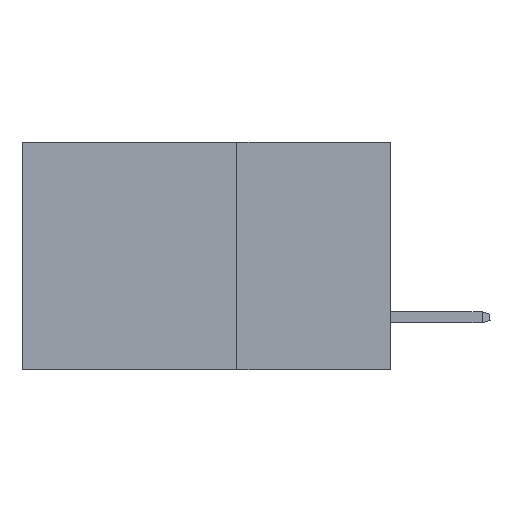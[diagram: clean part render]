
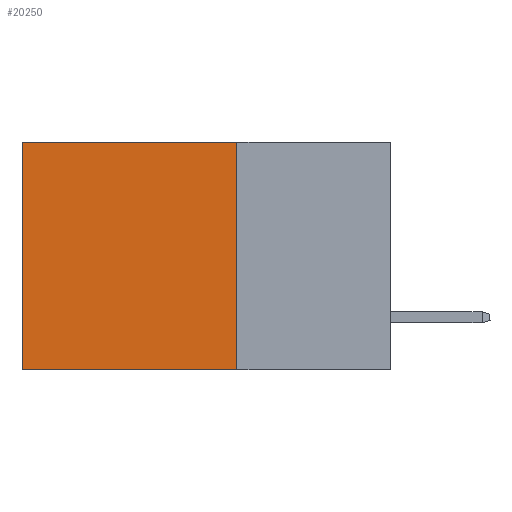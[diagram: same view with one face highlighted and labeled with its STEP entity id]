
A CAD part, left-side view. The second image highlights one B-rep face of the part: STEP entity #20250.
In plain terms, the highlighted planar face has unit normal (-1, 0, 0).
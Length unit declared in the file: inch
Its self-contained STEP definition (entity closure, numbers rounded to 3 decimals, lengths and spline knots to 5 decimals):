
#39 = ORIENTED_EDGE ( 'NONE', *, *, #12450, .F. ) ;
#1543 = CARTESIAN_POINT ( 'NONE',  ( 0.2875, 0.6, -0.37 ) ) ;
#7767 = LINE ( 'NONE', #8993, #19526 ) ;
#8753 = DIRECTION ( 'NONE',  ( 0., 0., -1. ) ) ;
#8993 = CARTESIAN_POINT ( 'NONE',  ( 0.2875, 0.25, 0. ) ) ;
#10341 = LINE ( 'NONE', #31055, #33421 ) ;
#11597 = ORIENTED_EDGE ( 'NONE', *, *, #26522, .T. ) ;
#12280 = DIRECTION ( 'NONE',  ( 0., 0., -1. ) ) ;
#12450 = EDGE_CURVE ( 'NONE', #19710, #16408, #22103, .T. ) ;
#13900 = CARTESIAN_POINT ( 'NONE',  ( 0.2875, 0.25, 0. ) ) ;
#15203 = PLANE ( 'NONE',  #25376 ) ;
#16408 = VERTEX_POINT ( 'NONE', #1543 ) ;
#16496 = VECTOR ( 'NONE', #16501, 39.37008 ) ;
#16501 = DIRECTION ( 'NONE',  ( 0., 1., 0. ) ) ;
#16559 = FACE_OUTER_BOUND ( 'NONE', #32175, .T. ) ;
#17199 = DIRECTION ( 'NONE',  ( 0., 1., 0. ) ) ;
#18089 = ORIENTED_EDGE ( 'NONE', *, *, #25509, .T. ) ;
#18432 = VERTEX_POINT ( 'NONE', #33924 ) ;
#19526 = VECTOR ( 'NONE', #8753, 39.37008 ) ;
#19710 = VERTEX_POINT ( 'NONE', #24877 ) ;
#19870 = LINE ( 'NONE', #28268, #25497 ) ;
#20250 = ADVANCED_FACE ( 'NONE', ( #16559 ), #15203, .F. ) ;
#21864 = VERTEX_POINT ( 'NONE', #13900 ) ;
#22103 = LINE ( 'NONE', #33255, #16496 ) ;
#24877 = CARTESIAN_POINT ( 'NONE',  ( 0.2875, 0.25, -0.37 ) ) ;
#25376 = AXIS2_PLACEMENT_3D ( 'NONE', #34766, #28936, #12280 ) ;
#25497 = VECTOR ( 'NONE', #30819, 39.37008 ) ;
#25509 = EDGE_CURVE ( 'NONE', #21864, #18432, #10341, .T. ) ;
#26522 = EDGE_CURVE ( 'NONE', #18432, #16408, #19870, .T. ) ;
#27327 = ORIENTED_EDGE ( 'NONE', *, *, #32774, .F. ) ;
#28268 = CARTESIAN_POINT ( 'NONE',  ( 0.2875, 0.6, 0. ) ) ;
#28936 = DIRECTION ( 'NONE',  ( 1., 0., 0. ) ) ;
#30819 = DIRECTION ( 'NONE',  ( 0., 0., -1. ) ) ;
#31055 = CARTESIAN_POINT ( 'NONE',  ( 0.2875, 0.25, 0. ) ) ;
#32175 = EDGE_LOOP ( 'NONE', ( #11597, #39, #27327, #18089 ) ) ;
#32774 = EDGE_CURVE ( 'NONE', #21864, #19710, #7767, .T. ) ;
#33255 = CARTESIAN_POINT ( 'NONE',  ( 0.2875, 0.25, -0.37 ) ) ;
#33421 = VECTOR ( 'NONE', #17199, 39.37008 ) ;
#33924 = CARTESIAN_POINT ( 'NONE',  ( 0.2875, 0.6, 0. ) ) ;
#34766 = CARTESIAN_POINT ( 'NONE',  ( 0.2875, 0.25, 0. ) ) ;
